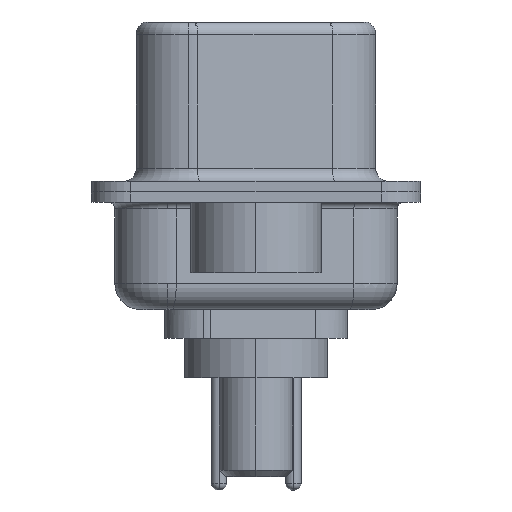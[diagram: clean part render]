
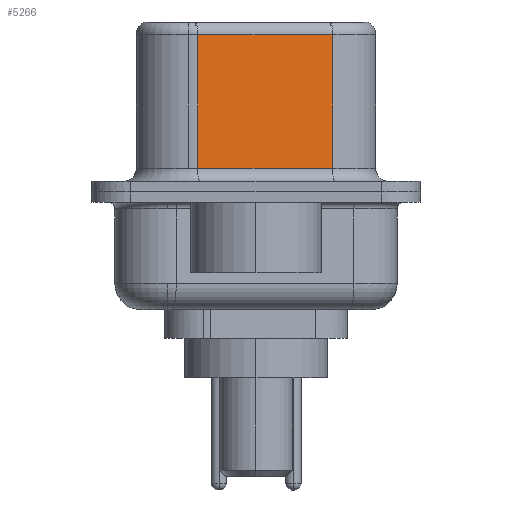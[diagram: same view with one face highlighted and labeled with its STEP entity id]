
A CAD part, left-side view. The second image highlights one B-rep face of the part: STEP entity #5266.
In plain terms, the highlighted planar face has unit normal (-0.985, -0.174, 0).
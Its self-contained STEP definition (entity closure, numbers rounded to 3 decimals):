
#1967 = VERTEX_POINT ( 'NONE', #2531 ) ;
#2531 = CARTESIAN_POINT ( 'NONE',  ( 4.58, -2.927, 6.02 ) ) ;
#3052 = CARTESIAN_POINT ( 'NONE',  ( 4.58, -2.927, 0.9 ) ) ;
#3540 = VECTOR ( 'NONE', #8107, 1000. ) ;
#4284 = CARTESIAN_POINT ( 'NONE',  ( 3.67, 2.233, 6.52 ) ) ;
#4484 = VERTEX_POINT ( 'NONE', #16674 ) ;
#5266 = ADVANCED_FACE ( 'NONE', ( #7658 ), #16429, .F. ) ;
#5279 = VECTOR ( 'NONE', #12942, 1000. ) ;
#5347 = EDGE_CURVE ( 'NONE', #1967, #10708, #20115, .T. ) ;
#6929 = DIRECTION ( 'NONE',  ( 0., 0., -1. ) ) ;
#7617 = DIRECTION ( 'NONE',  ( 0.985, 0.174, 0. ) ) ;
#7658 = FACE_OUTER_BOUND ( 'NONE', #12513, .T. ) ;
#7720 = VECTOR ( 'NONE', #6929, 1000. ) ;
#8107 = DIRECTION ( 'NONE',  ( 0., 0., -1. ) ) ;
#8594 = LINE ( 'NONE', #4284, #3540 ) ;
#8908 = CARTESIAN_POINT ( 'NONE',  ( 3.67, 2.233, 0.9 ) ) ;
#9086 = CARTESIAN_POINT ( 'NONE',  ( 4.58, -2.927, 6.02 ) ) ;
#9927 = CARTESIAN_POINT ( 'NONE',  ( 4.58, -2.927, 6.52 ) ) ;
#10351 = EDGE_CURVE ( 'NONE', #18203, #4484, #20229, .T. ) ;
#10451 = VECTOR ( 'NONE', #14297, 1000. ) ;
#10581 = ORIENTED_EDGE ( 'NONE', *, *, #5347, .T. ) ;
#10708 = VERTEX_POINT ( 'NONE', #19007 ) ;
#12099 = EDGE_CURVE ( 'NONE', #10708, #18203, #8594, .T. ) ;
#12122 = AXIS2_PLACEMENT_3D ( 'NONE', #9927, #7617, #13441 ) ;
#12513 = EDGE_LOOP ( 'NONE', ( #21809, #10581, #15990, #23271 ) ) ;
#12942 = DIRECTION ( 'NONE',  ( -0.174, 0.985, 0. ) ) ;
#13441 = DIRECTION ( 'NONE',  ( -0.174, 0.985, 0. ) ) ;
#14297 = DIRECTION ( 'NONE',  ( 0.174, -0.985, 0. ) ) ;
#15990 = ORIENTED_EDGE ( 'NONE', *, *, #12099, .T. ) ;
#16429 = PLANE ( 'NONE',  #12122 ) ;
#16674 = CARTESIAN_POINT ( 'NONE',  ( 4.58, -2.927, 0.9 ) ) ;
#17520 = LINE ( 'NONE', #19801, #7720 ) ;
#18203 = VERTEX_POINT ( 'NONE', #8908 ) ;
#18692 = EDGE_CURVE ( 'NONE', #1967, #4484, #17520, .T. ) ;
#19007 = CARTESIAN_POINT ( 'NONE',  ( 3.67, 2.233, 6.02 ) ) ;
#19801 = CARTESIAN_POINT ( 'NONE',  ( 4.58, -2.927, 6.52 ) ) ;
#20115 = LINE ( 'NONE', #9086, #5279 ) ;
#20229 = LINE ( 'NONE', #3052, #10451 ) ;
#21809 = ORIENTED_EDGE ( 'NONE', *, *, #18692, .F. ) ;
#23271 = ORIENTED_EDGE ( 'NONE', *, *, #10351, .T. ) ;
